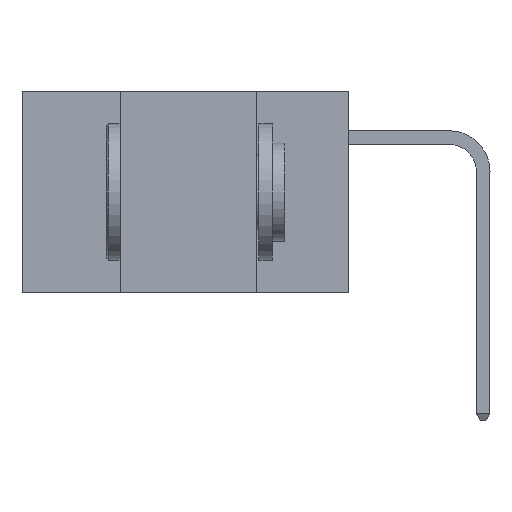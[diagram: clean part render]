
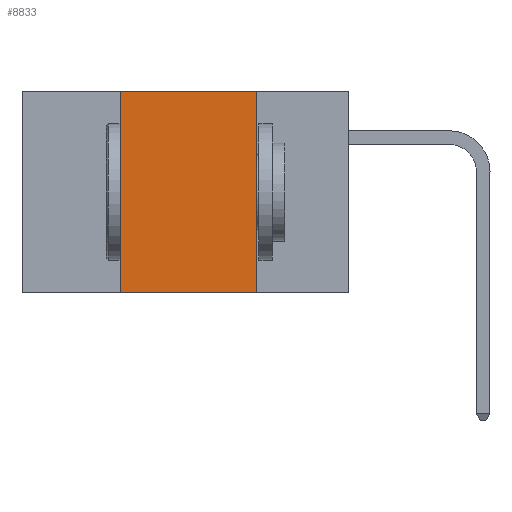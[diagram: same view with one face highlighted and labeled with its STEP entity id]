
A CAD part, left-side view. The second image highlights one B-rep face of the part: STEP entity #8833.
In plain terms, the highlighted planar face has unit normal (-1, 0, 0).
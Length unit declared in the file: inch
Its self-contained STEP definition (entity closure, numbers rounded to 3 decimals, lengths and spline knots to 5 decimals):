
#541 = DIRECTION ( 'NONE',  ( 0., -1., 0. ) ) ;
#673 = CARTESIAN_POINT ( 'NONE',  ( 0., 0.6, 0. ) ) ;
#702 = CARTESIAN_POINT ( 'NONE',  ( 0., 0.42, 0. ) ) ;
#769 = EDGE_CURVE ( 'NONE', #12983, #8849, #4782, .T. ) ;
#956 = ORIENTED_EDGE ( 'NONE', *, *, #769, .F. ) ;
#1121 = PLANE ( 'NONE',  #3531 ) ;
#1525 = EDGE_CURVE ( 'NONE', #3751, #12983, #6908, .T. ) ;
#1739 = FACE_OUTER_BOUND ( 'NONE', #6928, .T. ) ;
#2274 = DIRECTION ( 'NONE',  ( 1., 0., 0. ) ) ;
#3531 = AXIS2_PLACEMENT_3D ( 'NONE', #9098, #2274, #10289 ) ;
#3687 = DIRECTION ( 'NONE',  ( 0., 0., 1. ) ) ;
#3751 = VERTEX_POINT ( 'NONE', #10288 ) ;
#3870 = VECTOR ( 'NONE', #3687, 39.37008 ) ;
#4097 = CARTESIAN_POINT ( 'NONE',  ( 0., 0.42, 0. ) ) ;
#4782 = LINE ( 'NONE', #673, #8190 ) ;
#5143 = CARTESIAN_POINT ( 'NONE',  ( 0., 0.6, -0.37 ) ) ;
#5170 = LINE ( 'NONE', #5278, #10853 ) ;
#5278 = CARTESIAN_POINT ( 'NONE',  ( 0., 0.17, 0. ) ) ;
#5856 = VERTEX_POINT ( 'NONE', #14537 ) ;
#6177 = EDGE_CURVE ( 'NONE', #3751, #5856, #10613, .T. ) ;
#6268 = DIRECTION ( 'NONE',  ( 0., -1., 0. ) ) ;
#6908 = LINE ( 'NONE', #4097, #3870 ) ;
#6928 = EDGE_LOOP ( 'NONE', ( #13965, #956, #12857, #8646 ) ) ;
#8190 = VECTOR ( 'NONE', #541, 39.37008 ) ;
#8646 = ORIENTED_EDGE ( 'NONE', *, *, #6177, .T. ) ;
#8833 = ADVANCED_FACE ( 'NONE', ( #1739 ), #1121, .F. ) ;
#8849 = VERTEX_POINT ( 'NONE', #13515 ) ;
#9098 = CARTESIAN_POINT ( 'NONE',  ( 0., 0.6, 0. ) ) ;
#9234 = EDGE_CURVE ( 'NONE', #8849, #5856, #5170, .T. ) ;
#10288 = CARTESIAN_POINT ( 'NONE',  ( 0., 0.42, -0.37 ) ) ;
#10289 = DIRECTION ( 'NONE',  ( 0., 0., -1. ) ) ;
#10613 = LINE ( 'NONE', #5143, #13117 ) ;
#10853 = VECTOR ( 'NONE', #12022, 39.37008 ) ;
#12022 = DIRECTION ( 'NONE',  ( 0., 0., -1. ) ) ;
#12857 = ORIENTED_EDGE ( 'NONE', *, *, #1525, .F. ) ;
#12983 = VERTEX_POINT ( 'NONE', #702 ) ;
#13117 = VECTOR ( 'NONE', #6268, 39.37008 ) ;
#13515 = CARTESIAN_POINT ( 'NONE',  ( 0., 0.17, 0. ) ) ;
#13965 = ORIENTED_EDGE ( 'NONE', *, *, #9234, .F. ) ;
#14537 = CARTESIAN_POINT ( 'NONE',  ( 0., 0.17, -0.37 ) ) ;
